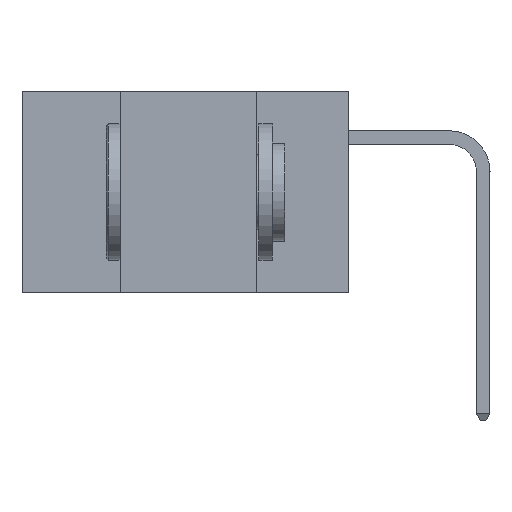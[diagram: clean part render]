
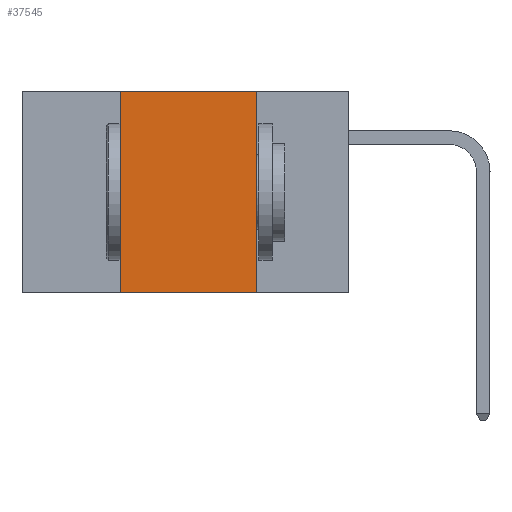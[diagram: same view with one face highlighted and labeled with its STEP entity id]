
A CAD part, left-side view. The second image highlights one B-rep face of the part: STEP entity #37545.
In plain terms, the highlighted planar face has unit normal (-1, 0, 0).
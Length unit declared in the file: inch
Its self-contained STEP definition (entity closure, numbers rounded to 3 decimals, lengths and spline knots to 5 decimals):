
#707 = CARTESIAN_POINT ( 'NONE',  ( 0., 0.6, 0. ) ) ;
#1483 = EDGE_CURVE ( 'NONE', #18187, #6650, #15058, .T. ) ;
#4223 = DIRECTION ( 'NONE',  ( 0., 0., -1. ) ) ;
#4796 = LINE ( 'NONE', #21064, #33207 ) ;
#5490 = DIRECTION ( 'NONE',  ( 0., -1., 0. ) ) ;
#6650 = VERTEX_POINT ( 'NONE', #23513 ) ;
#6865 = VERTEX_POINT ( 'NONE', #23176 ) ;
#9650 = DIRECTION ( 'NONE',  ( 0., 0., 1. ) ) ;
#14596 = VECTOR ( 'NONE', #9650, 39.37008 ) ;
#15058 = LINE ( 'NONE', #18020, #14596 ) ;
#16289 = CARTESIAN_POINT ( 'NONE',  ( 0., 0.6, 0. ) ) ;
#16362 = CARTESIAN_POINT ( 'NONE',  ( 0., 0.17, 0. ) ) ;
#18020 = CARTESIAN_POINT ( 'NONE',  ( 0., 0.42, 0. ) ) ;
#18187 = VERTEX_POINT ( 'NONE', #21471 ) ;
#18467 = ORIENTED_EDGE ( 'NONE', *, *, #25124, .T. ) ;
#18919 = EDGE_CURVE ( 'NONE', #20808, #6865, #32661, .T. ) ;
#18943 = LINE ( 'NONE', #707, #35986 ) ;
#20470 = AXIS2_PLACEMENT_3D ( 'NONE', #16289, #36925, #4223 ) ;
#20808 = VERTEX_POINT ( 'NONE', #16362 ) ;
#21064 = CARTESIAN_POINT ( 'NONE',  ( 0., 0.6, -0.37 ) ) ;
#21471 = CARTESIAN_POINT ( 'NONE',  ( 0., 0.42, -0.37 ) ) ;
#21826 = PLANE ( 'NONE',  #20470 ) ;
#21921 = DIRECTION ( 'NONE',  ( 0., 0., -1. ) ) ;
#23176 = CARTESIAN_POINT ( 'NONE',  ( 0., 0.17, -0.37 ) ) ;
#23513 = CARTESIAN_POINT ( 'NONE',  ( 0., 0.42, 0. ) ) ;
#25124 = EDGE_CURVE ( 'NONE', #18187, #6865, #4796, .T. ) ;
#26891 = ORIENTED_EDGE ( 'NONE', *, *, #32537, .F. ) ;
#26983 = VECTOR ( 'NONE', #21921, 39.37008 ) ;
#28117 = DIRECTION ( 'NONE',  ( 0., -1., 0. ) ) ;
#29477 = ORIENTED_EDGE ( 'NONE', *, *, #18919, .F. ) ;
#32537 = EDGE_CURVE ( 'NONE', #6650, #20808, #18943, .T. ) ;
#32661 = LINE ( 'NONE', #33584, #26983 ) ;
#33198 = ORIENTED_EDGE ( 'NONE', *, *, #1483, .F. ) ;
#33207 = VECTOR ( 'NONE', #5490, 39.37008 ) ;
#33584 = CARTESIAN_POINT ( 'NONE',  ( 0., 0.17, 0. ) ) ;
#35076 = FACE_OUTER_BOUND ( 'NONE', #35095, .T. ) ;
#35095 = EDGE_LOOP ( 'NONE', ( #29477, #26891, #33198, #18467 ) ) ;
#35986 = VECTOR ( 'NONE', #28117, 39.37008 ) ;
#36925 = DIRECTION ( 'NONE',  ( 1., 0., 0. ) ) ;
#37545 = ADVANCED_FACE ( 'NONE', ( #35076 ), #21826, .F. ) ;
